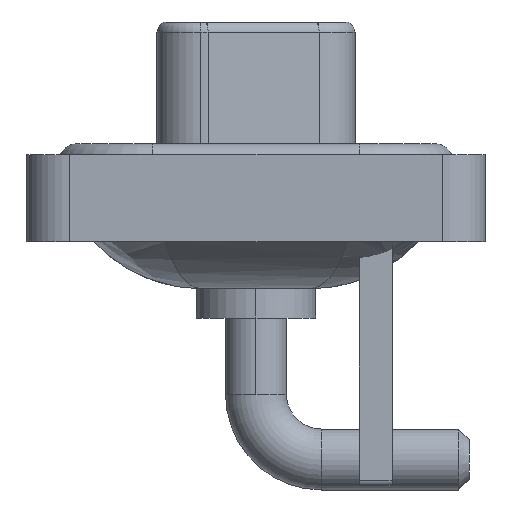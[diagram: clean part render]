
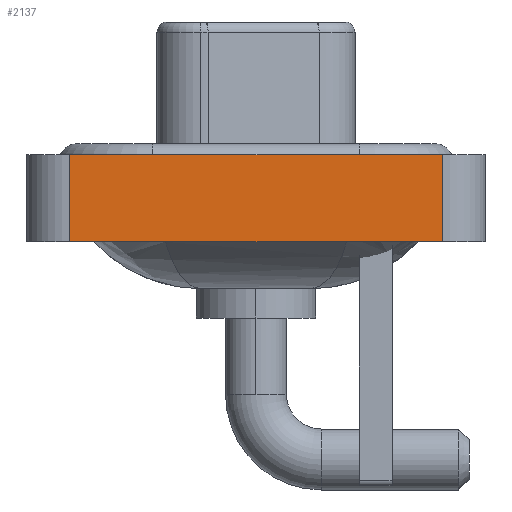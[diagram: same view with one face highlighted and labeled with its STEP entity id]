
A CAD part, left-side view. The second image highlights one B-rep face of the part: STEP entity #2137.
In plain terms, the highlighted planar face has unit normal (-1, 0, 0).
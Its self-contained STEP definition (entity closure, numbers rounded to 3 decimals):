
#464 = CARTESIAN_POINT ( 'NONE',  ( -7.35, -8.55, -3.6 ) ) ;
#539 = LINE ( 'NONE', #14846, #12933 ) ;
#761 = VECTOR ( 'NONE', #10005, 1000. ) ;
#2137 = ADVANCED_FACE ( 'NONE', ( #3262 ), #9245, .T. ) ;
#2373 = CARTESIAN_POINT ( 'NONE',  ( -7.35, 8.55, -3.6 ) ) ;
#3262 = FACE_OUTER_BOUND ( 'NONE', #10140, .T. ) ;
#3983 = EDGE_CURVE ( 'NONE', #17183, #6656, #539, .T. ) ;
#4273 = CARTESIAN_POINT ( 'NONE',  ( -7.35, -8.55, -3.6 ) ) ;
#4430 = AXIS2_PLACEMENT_3D ( 'NONE', #464, #17725, #14956 ) ;
#5393 = DIRECTION ( 'NONE',  ( 0., -1., 0. ) ) ;
#5984 = LINE ( 'NONE', #4273, #18407 ) ;
#6656 = VERTEX_POINT ( 'NONE', #6700 ) ;
#6700 = CARTESIAN_POINT ( 'NONE',  ( -7.35, 8.55, 0.4 ) ) ;
#6797 = CARTESIAN_POINT ( 'NONE',  ( -7.35, -8.55, 0.4 ) ) ;
#7237 = ORIENTED_EDGE ( 'NONE', *, *, #3983, .F. ) ;
#8669 = EDGE_CURVE ( 'NONE', #17183, #18138, #11423, .T. ) ;
#9245 = PLANE ( 'NONE',  #4430 ) ;
#9610 = ORIENTED_EDGE ( 'NONE', *, *, #8669, .T. ) ;
#9840 = CARTESIAN_POINT ( 'NONE',  ( -7.35, -8.55, -3.6 ) ) ;
#10005 = DIRECTION ( 'NONE',  ( 0., -1., 0. ) ) ;
#10140 = EDGE_LOOP ( 'NONE', ( #14594, #11335, #7237, #9610 ) ) ;
#11335 = ORIENTED_EDGE ( 'NONE', *, *, #18192, .F. ) ;
#11423 = LINE ( 'NONE', #15890, #761 ) ;
#12888 = VERTEX_POINT ( 'NONE', #17817 ) ;
#12933 = VECTOR ( 'NONE', #13426, 1000. ) ;
#13400 = DIRECTION ( 'NONE',  ( 0., 0., 1. ) ) ;
#13426 = DIRECTION ( 'NONE',  ( 0., 0., 1. ) ) ;
#14457 = VECTOR ( 'NONE', #5393, 1000. ) ;
#14594 = ORIENTED_EDGE ( 'NONE', *, *, #15904, .T. ) ;
#14846 = CARTESIAN_POINT ( 'NONE',  ( -7.35, 8.55, -3.6 ) ) ;
#14956 = DIRECTION ( 'NONE',  ( 0., 0., 1. ) ) ;
#15890 = CARTESIAN_POINT ( 'NONE',  ( -7.35, -8.55, -3.6 ) ) ;
#15904 = EDGE_CURVE ( 'NONE', #18138, #12888, #5984, .T. ) ;
#17069 = LINE ( 'NONE', #6797, #14457 ) ;
#17183 = VERTEX_POINT ( 'NONE', #2373 ) ;
#17725 = DIRECTION ( 'NONE',  ( -1., 0., 0. ) ) ;
#17817 = CARTESIAN_POINT ( 'NONE',  ( -7.35, -8.55, 0.4 ) ) ;
#18138 = VERTEX_POINT ( 'NONE', #9840 ) ;
#18192 = EDGE_CURVE ( 'NONE', #6656, #12888, #17069, .T. ) ;
#18407 = VECTOR ( 'NONE', #13400, 1000. ) ;
